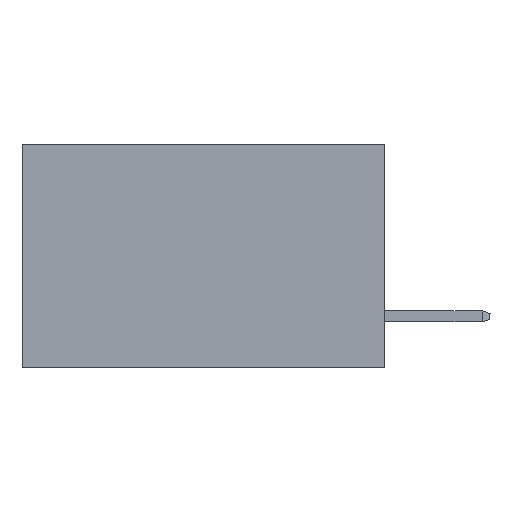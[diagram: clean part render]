
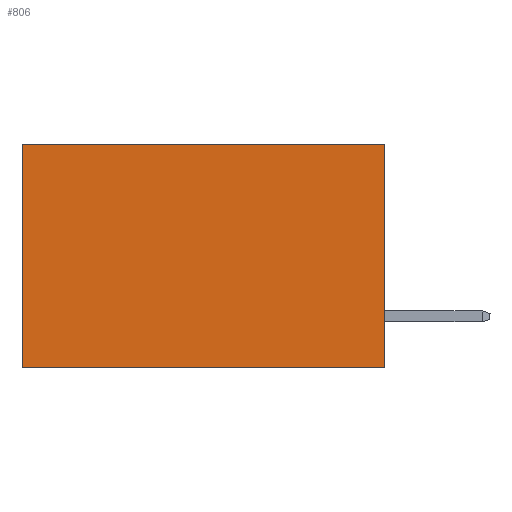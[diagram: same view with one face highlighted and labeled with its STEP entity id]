
A CAD part, left-side view. The second image highlights one B-rep face of the part: STEP entity #806.
In plain terms, the highlighted planar face has unit normal (-1, 0, 0).
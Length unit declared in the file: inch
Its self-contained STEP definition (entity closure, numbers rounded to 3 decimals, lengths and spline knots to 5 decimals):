
#59 = ORIENTED_EDGE ( 'NONE', *, *, #12053, .F. ) ;
#106 = CARTESIAN_POINT ( 'NONE',  ( 0.2615, 0., 0. ) ) ;
#296 = LINE ( 'NONE', #1342, #8617 ) ;
#806 = ADVANCED_FACE ( 'NONE', ( #14276 ), #10868, .F. ) ;
#876 = CARTESIAN_POINT ( 'NONE',  ( 0.2615, 0., -0.37 ) ) ;
#1342 = CARTESIAN_POINT ( 'NONE',  ( 0.2615, 0., -0.37 ) ) ;
#1483 = EDGE_CURVE ( 'NONE', #12577, #13731, #13243, .T. ) ;
#1657 = CARTESIAN_POINT ( 'NONE',  ( 0.2615, 0.6, -0.37 ) ) ;
#1681 = EDGE_LOOP ( 'NONE', ( #10222, #59, #10791, #3247 ) ) ;
#2503 = DIRECTION ( 'NONE',  ( 0., 1., 0. ) ) ;
#2828 = CARTESIAN_POINT ( 'NONE',  ( 0.2615, 0., 0. ) ) ;
#3247 = ORIENTED_EDGE ( 'NONE', *, *, #14038, .T. ) ;
#3259 = DIRECTION ( 'NONE',  ( 0., 0., -1. ) ) ;
#4306 = DIRECTION ( 'NONE',  ( 0., 0., -1. ) ) ;
#5441 = DIRECTION ( 'NONE',  ( 0., 0., -1. ) ) ;
#5517 = EDGE_CURVE ( 'NONE', #6182, #12520, #8785, .T. ) ;
#6182 = VERTEX_POINT ( 'NONE', #8106 ) ;
#6189 = VECTOR ( 'NONE', #5441, 39.37008 ) ;
#6768 = DIRECTION ( 'NONE',  ( 0., 1., 0. ) ) ;
#7561 = CARTESIAN_POINT ( 'NONE',  ( 0.2615, 0., -0.37 ) ) ;
#8106 = CARTESIAN_POINT ( 'NONE',  ( 0.2615, 0.6, 0. ) ) ;
#8230 = VECTOR ( 'NONE', #3259, 39.37008 ) ;
#8617 = VECTOR ( 'NONE', #2503, 39.37008 ) ;
#8785 = LINE ( 'NONE', #10837, #6189 ) ;
#9308 = CARTESIAN_POINT ( 'NONE',  ( 0.2615, 0., -0.37 ) ) ;
#9764 = DIRECTION ( 'NONE',  ( 1., 0., 0. ) ) ;
#9962 = VECTOR ( 'NONE', #6768, 39.37008 ) ;
#10222 = ORIENTED_EDGE ( 'NONE', *, *, #5517, .T. ) ;
#10517 = AXIS2_PLACEMENT_3D ( 'NONE', #876, #9764, #4306 ) ;
#10791 = ORIENTED_EDGE ( 'NONE', *, *, #1483, .F. ) ;
#10837 = CARTESIAN_POINT ( 'NONE',  ( 0.2615, 0.6, -0.37 ) ) ;
#10868 = PLANE ( 'NONE',  #10517 ) ;
#11568 = LINE ( 'NONE', #106, #9962 ) ;
#12053 = EDGE_CURVE ( 'NONE', #13731, #12520, #296, .T. ) ;
#12520 = VERTEX_POINT ( 'NONE', #1657 ) ;
#12577 = VERTEX_POINT ( 'NONE', #2828 ) ;
#13243 = LINE ( 'NONE', #7561, #8230 ) ;
#13731 = VERTEX_POINT ( 'NONE', #9308 ) ;
#14038 = EDGE_CURVE ( 'NONE', #12577, #6182, #11568, .T. ) ;
#14276 = FACE_OUTER_BOUND ( 'NONE', #1681, .T. ) ;
